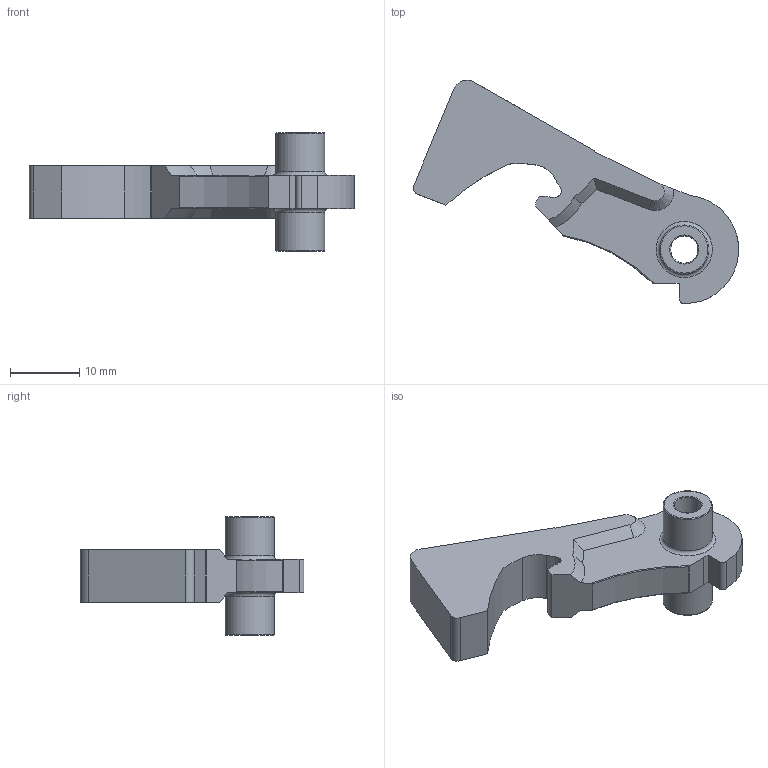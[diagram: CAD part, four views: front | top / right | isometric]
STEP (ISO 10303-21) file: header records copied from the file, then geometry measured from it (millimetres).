
FILE_DESCRIPTION(/* description */ (''),/* implementation_level */ '2;1');
FILE_NAME(/* name */ 'Hammer.step',/* time_stamp */ '2022-05-12T09:39:13-06:00',/* author */ (''),/* organization */ (''),/* preprocessor_version */ 'ST-DEVELOPER v18.1',/* originating_system */ 'Autodesk Translation Framework v10.10.0.1391',/* authorisation */ '');
FILE_SCHEMA (('AUTOMOTIVE_DESIGN { 1 0 10303 214 3 1 1 }'));
Length unit declared in the file: millimetre
Products named in the file (1): Hammer
Bounding box: 47.08 x 32.4 x 17.17 mm (x, y, z)
Volume: 3690.8 mm3; surface area: 2713.4 mm2
Topology: 1 solids, 1 shells, 68 faces, 179 edges, 117 vertices
Faces by surface type: cylinder 25, plane 23, torus 10, cone 6, bspline 4
Full cylindrical faces by diameter (mm): 0.813 x1, 3.9 x1, 3.962 x1, 7.112 x2, 7.366 x1
Entity records: 2394 total; most frequent: CARTESIAN_POINT 626, DIRECTION 379, ORIENTED_EDGE 358, EDGE_CURVE 179, AXIS2_PLACEMENT_3D 151, VERTEX_POINT 117, CIRCLE 80, LINE 77
